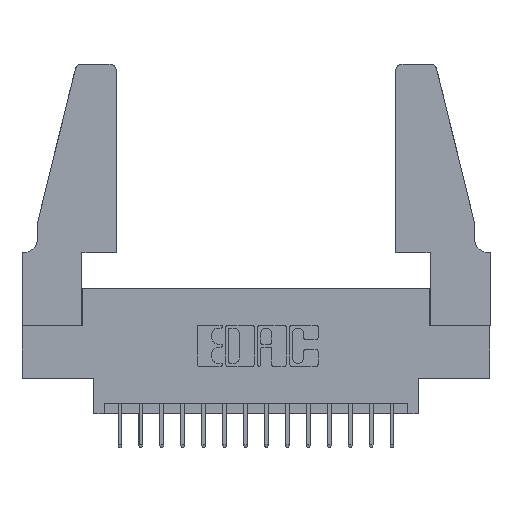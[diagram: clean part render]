
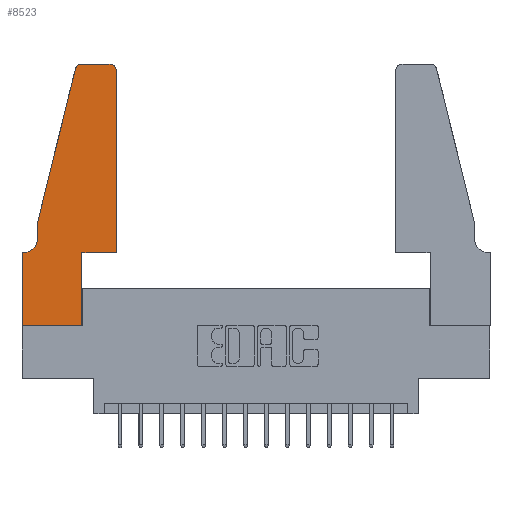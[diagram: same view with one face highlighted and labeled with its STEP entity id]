
A CAD part, top view. The second image highlights one B-rep face of the part: STEP entity #8523.
In plain terms, the highlighted planar face has unit normal (0, 0, 1).
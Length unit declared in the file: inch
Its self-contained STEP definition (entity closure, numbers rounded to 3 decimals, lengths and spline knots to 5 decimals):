
#410 = CARTESIAN_POINT ( 'NONE',  ( 0., 0., 0.37 ) ) ;
#580 = VERTEX_POINT ( 'NONE', #410 ) ;
#587 = ORIENTED_EDGE ( 'NONE', *, *, #9942, .T. ) ;
#662 = CARTESIAN_POINT ( 'NONE',  ( 0.4505, 0.35, 0.37 ) ) ;
#847 = CARTESIAN_POINT ( 'NONE',  ( 0.0055, 0.42, 0.37 ) ) ;
#1525 = EDGE_CURVE ( 'NONE', #10268, #7187, #11822, .T. ) ;
#1737 = DIRECTION ( 'NONE',  ( 0., 0., 1. ) ) ;
#2282 = DIRECTION ( 'NONE',  ( -1., 0., 0. ) ) ;
#2443 = CARTESIAN_POINT ( 'NONE',  ( 0., 0., 0.37 ) ) ;
#2849 = VERTEX_POINT ( 'NONE', #8264 ) ;
#2886 = CARTESIAN_POINT ( 'NONE',  ( 0.4505, 0.35, 0.37 ) ) ;
#2914 = VECTOR ( 'NONE', #5197, 39.37008 ) ;
#2983 = CARTESIAN_POINT ( 'NONE',  ( 0.0055, 0.35, 0.37 ) ) ;
#3096 = ORIENTED_EDGE ( 'NONE', *, *, #7449, .T. ) ;
#3139 = CARTESIAN_POINT ( 'NONE',  ( 0.25487, 1.22718, 0.37 ) ) ;
#3421 = CARTESIAN_POINT ( 'NONE',  ( 0., 0., 0.37 ) ) ;
#3516 = DIRECTION ( 'NONE',  ( -1., 0., 0. ) ) ;
#3676 = AXIS2_PLACEMENT_3D ( 'NONE', #6990, #4465, #13515 ) ;
#3740 = VECTOR ( 'NONE', #4279, 39.37008 ) ;
#3970 = ORIENTED_EDGE ( 'NONE', *, *, #14580, .T. ) ;
#4208 = LINE ( 'NONE', #9907, #14561 ) ;
#4279 = DIRECTION ( 'NONE',  ( 0., 1., 0. ) ) ;
#4355 = CARTESIAN_POINT ( 'NONE',  ( 0.4505, 0.35, 0.37 ) ) ;
#4465 = DIRECTION ( 'NONE',  ( 0., 0., 1. ) ) ;
#4601 = VECTOR ( 'NONE', #3516, 39.37008 ) ;
#4642 = CARTESIAN_POINT ( 'NONE',  ( 0.0755, 0.5, 0.37 ) ) ;
#4857 = CARTESIAN_POINT ( 'NONE',  ( 0.284, 1.25, 0.37 ) ) ;
#4872 = EDGE_CURVE ( 'NONE', #8358, #7312, #12771, .T. ) ;
#5197 = DIRECTION ( 'NONE',  ( 0., -1., 0. ) ) ;
#5336 = VECTOR ( 'NONE', #11188, 39.37008 ) ;
#5616 = ORIENTED_EDGE ( 'NONE', *, *, #10138, .T. ) ;
#5932 = VERTEX_POINT ( 'NONE', #2983 ) ;
#6210 = VECTOR ( 'NONE', #16252, 39.37008 ) ;
#6359 = EDGE_CURVE ( 'NONE', #16838, #580, #9867, .T. ) ;
#6376 = ORIENTED_EDGE ( 'NONE', *, *, #6359, .T. ) ;
#6532 = VERTEX_POINT ( 'NONE', #14609 ) ;
#6692 = AXIS2_PLACEMENT_3D ( 'NONE', #9672, #1737, #10963 ) ;
#6971 = ORIENTED_EDGE ( 'NONE', *, *, #10260, .T. ) ;
#6990 = CARTESIAN_POINT ( 'NONE',  ( 0., 0.35, 0.37 ) ) ;
#7026 = VECTOR ( 'NONE', #10016, 39.37008 ) ;
#7187 = VERTEX_POINT ( 'NONE', #3139 ) ;
#7312 = VERTEX_POINT ( 'NONE', #15034 ) ;
#7449 = EDGE_CURVE ( 'NONE', #6532, #5932, #12587, .T. ) ;
#7669 = FACE_OUTER_BOUND ( 'NONE', #10256, .T. ) ;
#8264 = CARTESIAN_POINT ( 'NONE',  ( 0.2865, 0.35, 0.37 ) ) ;
#8358 = VERTEX_POINT ( 'NONE', #11847 ) ;
#8523 = ADVANCED_FACE ( 'NONE', ( #7669 ), #12204, .T. ) ;
#8660 = EDGE_CURVE ( 'NONE', #5932, #16838, #12136, .T. ) ;
#8682 = CARTESIAN_POINT ( 'NONE',  ( 0.2605, 1.25, 0.37 ) ) ;
#9042 = ORIENTED_EDGE ( 'NONE', *, *, #1525, .T. ) ;
#9173 = DIRECTION ( 'NONE',  ( -1., 0., 0. ) ) ;
#9176 = ORIENTED_EDGE ( 'NONE', *, *, #4872, .T. ) ;
#9382 = ORIENTED_EDGE ( 'NONE', *, *, #10772, .T. ) ;
#9437 = VECTOR ( 'NONE', #10588, 39.37008 ) ;
#9642 = LINE ( 'NONE', #10993, #6210 ) ;
#9672 = CARTESIAN_POINT ( 'NONE',  ( 0.4205, 1.22, 0.37 ) ) ;
#9844 = DIRECTION ( 'NONE',  ( 0., 0., 1. ) ) ;
#9847 = DIRECTION ( 'NONE',  ( 0., -1., 0. ) ) ;
#9867 = LINE ( 'NONE', #2443, #2914 ) ;
#9907 = CARTESIAN_POINT ( 'NONE',  ( 0.0755, 0.5, 0.37 ) ) ;
#9942 = EDGE_CURVE ( 'NONE', #16648, #2849, #12898, .T. ) ;
#10016 = DIRECTION ( 'NONE',  ( 1., 0., 0. ) ) ;
#10052 = ORIENTED_EDGE ( 'NONE', *, *, #11446, .T. ) ;
#10138 = EDGE_CURVE ( 'NONE', #7187, #15735, #9642, .T. ) ;
#10169 = DIRECTION ( 'NONE',  ( 0., 0., -1. ) ) ;
#10256 = EDGE_LOOP ( 'NONE', ( #6971, #9042, #5616, #3970, #3096, #17106, #6376, #12453, #587, #9382, #10052, #9176 ) ) ;
#10260 = EDGE_CURVE ( 'NONE', #7312, #10268, #14942, .T. ) ;
#10268 = VERTEX_POINT ( 'NONE', #4857 ) ;
#10384 = DIRECTION ( 'NONE',  ( 1., 0., 0. ) ) ;
#10588 = DIRECTION ( 'NONE',  ( 0., 1., 0. ) ) ;
#10772 = EDGE_CURVE ( 'NONE', #2849, #12637, #14339, .T. ) ;
#10963 = DIRECTION ( 'NONE',  ( 1., 0., 0. ) ) ;
#10993 = CARTESIAN_POINT ( 'NONE',  ( 0.0755, 0.5, 0.37 ) ) ;
#11188 = DIRECTION ( 'NONE',  ( 1., 0., 0. ) ) ;
#11446 = EDGE_CURVE ( 'NONE', #12637, #8358, #14113, .T. ) ;
#11822 = CIRCLE ( 'NONE', #15235, 0.03 ) ;
#11847 = CARTESIAN_POINT ( 'NONE',  ( 0.4505, 1.22, 0.37 ) ) ;
#12136 = LINE ( 'NONE', #13039, #15598 ) ;
#12204 = PLANE ( 'NONE',  #3676 ) ;
#12211 = LINE ( 'NONE', #3421, #5336 ) ;
#12453 = ORIENTED_EDGE ( 'NONE', *, *, #17085, .T. ) ;
#12587 = CIRCLE ( 'NONE', #12798, 0.07 ) ;
#12637 = VERTEX_POINT ( 'NONE', #4355 ) ;
#12771 = CIRCLE ( 'NONE', #6692, 0.03 ) ;
#12798 = AXIS2_PLACEMENT_3D ( 'NONE', #847, #10169, #2282 ) ;
#12898 = LINE ( 'NONE', #14502, #9437 ) ;
#13039 = CARTESIAN_POINT ( 'NONE',  ( 0.0755, 0.35, 0.37 ) ) ;
#13515 = DIRECTION ( 'NONE',  ( 1., 0., 0. ) ) ;
#14113 = LINE ( 'NONE', #2886, #3740 ) ;
#14339 = LINE ( 'NONE', #662, #7026 ) ;
#14502 = CARTESIAN_POINT ( 'NONE',  ( 0.2865, 0.35, 0.37 ) ) ;
#14561 = VECTOR ( 'NONE', #9847, 39.37008 ) ;
#14580 = EDGE_CURVE ( 'NONE', #15735, #6532, #4208, .T. ) ;
#14609 = CARTESIAN_POINT ( 'NONE',  ( 0.0755, 0.42, 0.37 ) ) ;
#14637 = CARTESIAN_POINT ( 'NONE',  ( 0., 0.35, 0.37 ) ) ;
#14942 = LINE ( 'NONE', #8682, #4601 ) ;
#15034 = CARTESIAN_POINT ( 'NONE',  ( 0.4205, 1.25, 0.37 ) ) ;
#15235 = AXIS2_PLACEMENT_3D ( 'NONE', #16885, #9844, #10384 ) ;
#15533 = CARTESIAN_POINT ( 'NONE',  ( 0.2865, 0., 0.37 ) ) ;
#15598 = VECTOR ( 'NONE', #9173, 39.37008 ) ;
#15735 = VERTEX_POINT ( 'NONE', #4642 ) ;
#16252 = DIRECTION ( 'NONE',  ( -0.239, -0.971, 0. ) ) ;
#16648 = VERTEX_POINT ( 'NONE', #15533 ) ;
#16838 = VERTEX_POINT ( 'NONE', #14637 ) ;
#16885 = CARTESIAN_POINT ( 'NONE',  ( 0.284, 1.22, 0.37 ) ) ;
#17085 = EDGE_CURVE ( 'NONE', #580, #16648, #12211, .T. ) ;
#17106 = ORIENTED_EDGE ( 'NONE', *, *, #8660, .T. ) ;
